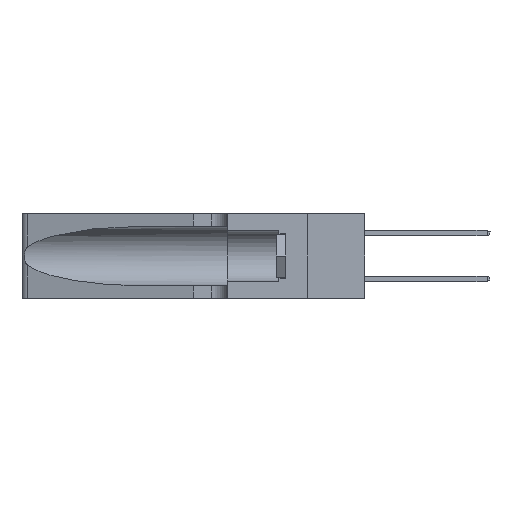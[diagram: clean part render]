
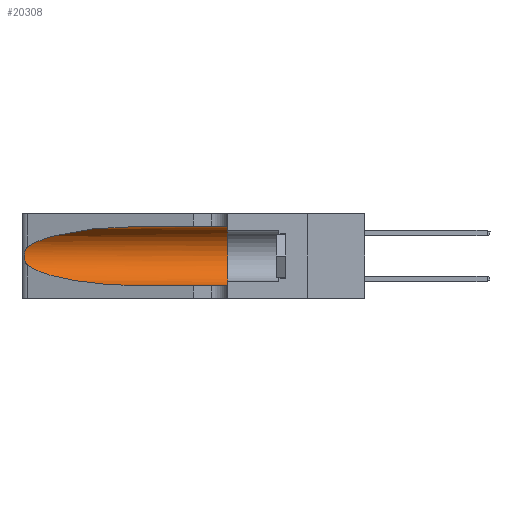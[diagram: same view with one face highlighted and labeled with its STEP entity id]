
A CAD part, left-side view. The second image highlights one B-rep face of the part: STEP entity #20308.
In plain terms, the highlighted cylindrical face has radius 3.308 mm (diameter 6.617 mm), a partial arc.
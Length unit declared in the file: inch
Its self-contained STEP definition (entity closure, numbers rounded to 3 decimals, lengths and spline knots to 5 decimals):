
#182 = CARTESIAN_POINT ( 'NONE',  ( 0.25639, 1.23184, 0.21858 ) ) ;
#560 = DIRECTION ( 'NONE',  ( 0., -1., 0. ) ) ;
#1215 = EDGE_CURVE ( 'NONE', #14818, #31055, #26149, .T. ) ;
#1867 = CARTESIAN_POINT ( 'NONE',  ( 0.1305, 0.72297, 0.05475 ) ) ;
#2061 = ORIENTED_EDGE ( 'NONE', *, *, #29288, .T. ) ;
#2638 = CARTESIAN_POINT ( 'NONE',  ( 0.25856, 1.23593, 0.16098 ) ) ;
#3086 = CARTESIAN_POINT ( 'NONE',  ( 0.1305, 0.72297, 0.05475 ) ) ;
#3107 = EDGE_CURVE ( 'NONE', #6114, #22241, #11570, .T. ) ;
#3572 = EDGE_LOOP ( 'NONE', ( #2061, #31905, #7103, #6359, #7499, #11759 ) ) ;
#5109 = CARTESIAN_POINT ( 'NONE',  ( 0.25555, 1.22993, 0.14849 ) ) ;
#5415 = CARTESIAN_POINT ( 'NONE',  ( 0.25487, 1.22718, 0.22369 ) ) ;
#5773 = EDGE_CURVE ( 'NONE', #16697, #6114, #20204, .T. ) ;
#5840 = FACE_OUTER_BOUND ( 'NONE', #3572, .T. ) ;
#6114 = VERTEX_POINT ( 'NONE', #25859 ) ;
#6311 = AXIS2_PLACEMENT_3D ( 'NONE', #24553, #15568, #17398 ) ;
#6359 = ORIENTED_EDGE ( 'NONE', *, *, #10248, .T. ) ;
#6802 = CARTESIAN_POINT ( 'NONE',  ( 0.1305, 0.72297, 0.31525 ) ) ;
#7103 = ORIENTED_EDGE ( 'NONE', *, *, #3107, .T. ) ;
#7499 = ORIENTED_EDGE ( 'NONE', *, *, #1215, .F. ) ;
#7615 = CARTESIAN_POINT ( 'NONE',  ( 0.25487, 1.22718, 0.14631 ) ) ;
#10207 = CARTESIAN_POINT ( 'NONE',  ( 0.1305, 0.35, 0.05475 ) ) ;
#10248 = EDGE_CURVE ( 'NONE', #22241, #31055, #28049, .T. ) ;
#10265 = CARTESIAN_POINT ( 'NONE',  ( 0.25787, 1.23484, 0.2124 ) ) ;
#10370 = CARTESIAN_POINT ( 'NONE',  ( 0.26075, 1.23896, 0.178 ) ) ;
#10415 = CARTESIAN_POINT ( 'NONE',  ( 0.1305, 0.72297, 0.31525 ) ) ;
#10832 = LINE ( 'NONE', #13184, #22424 ) ;
#11570 =( BOUNDED_CURVE ( )  B_SPLINE_CURVE ( 3, ( #19028, #19250, #26497, #1867 ),
 .UNSPECIFIED., .F., .F. ) 
 B_SPLINE_CURVE_WITH_KNOTS ( ( 4, 4 ),
 ( 3.44316, 4.71239 ),
 .UNSPECIFIED. ) 
 CURVE ( )  GEOMETRIC_REPRESENTATION_ITEM ( )  RATIONAL_B_SPLINE_CURVE ( ( 1., 0.87, 0.87, 1. ) ) 
 REPRESENTATION_ITEM ( '' )  );
#11759 = ORIENTED_EDGE ( 'NONE', *, *, #20320, .F. ) ;
#12195 = DIRECTION ( 'NONE',  ( 0., 1., 0. ) ) ;
#12853 = CARTESIAN_POINT ( 'NONE',  ( 0.1305, 1.61858, 0.05475 ) ) ;
#13184 = CARTESIAN_POINT ( 'NONE',  ( 0.1305, 1.61858, 0.31525 ) ) ;
#13583 = AXIS2_PLACEMENT_3D ( 'NONE', #14781, #12195, #29598 ) ;
#14527 =( BOUNDED_CURVE ( )  B_SPLINE_CURVE ( 3, ( #10415, #22418, #28750, #14672 ),
 .UNSPECIFIED., .F., .F. ) 
 B_SPLINE_CURVE_WITH_KNOTS ( ( 4, 4 ),
 ( 1.5708, 2.84003 ),
 .UNSPECIFIED. ) 
 CURVE ( )  GEOMETRIC_REPRESENTATION_ITEM ( )  RATIONAL_B_SPLINE_CURVE ( ( 1., 0.87, 0.87, 1. ) ) 
 REPRESENTATION_ITEM ( '' )  );
#14672 = CARTESIAN_POINT ( 'NONE',  ( 0.25487, 1.22718, 0.22369 ) ) ;
#14781 = CARTESIAN_POINT ( 'NONE',  ( 0.1305, 0.35, 0.185 ) ) ;
#14818 = VERTEX_POINT ( 'NONE', #25542 ) ;
#15047 = CARTESIAN_POINT ( 'NONE',  ( 0.25854, 1.2359, 0.20912 ) ) ;
#15568 = DIRECTION ( 'NONE',  ( 0., -1., 0. ) ) ;
#16697 = VERTEX_POINT ( 'NONE', #29716 ) ;
#17398 = DIRECTION ( 'NONE',  ( 0., 0., -1. ) ) ;
#17439 = CARTESIAN_POINT ( 'NONE',  ( 0.26018, 1.23835, 0.19895 ) ) ;
#17639 = CARTESIAN_POINT ( 'NONE',  ( 0.26075, 1.23896, 0.19203 ) ) ;
#17830 = DIRECTION ( 'NONE',  ( 0., -1., 0. ) ) ;
#19028 = CARTESIAN_POINT ( 'NONE',  ( 0.25487, 1.22718, 0.14631 ) ) ;
#19250 = CARTESIAN_POINT ( 'NONE',  ( 0.2373, 1.15595, 0.08982 ) ) ;
#20125 = CARTESIAN_POINT ( 'NONE',  ( 0.25789, 1.23486, 0.15765 ) ) ;
#20204 = B_SPLINE_CURVE_WITH_KNOTS ( 'NONE', 3,
 ( #5415, #22681, #182, #10265, #15047, #17439, #17639, #10370, #24993, #2638, #20125, #27611, #5109, #7615 ),
 .UNSPECIFIED., .F., .F.,
 ( 4, 2, 2, 2, 2, 2, 4 ),
 ( 0., 0.00027, 0.00053, 0.00107, 0.0016, 0.00187, 0.00214 ),
 .UNSPECIFIED. ) ;
#20308 = ADVANCED_FACE ( 'NONE', ( #5840 ), #28262, .F. ) ;
#20320 = EDGE_CURVE ( 'NONE', #25847, #14818, #10832, .T. ) ;
#22241 = VERTEX_POINT ( 'NONE', #3086 ) ;
#22418 = CARTESIAN_POINT ( 'NONE',  ( 0.18966, 0.96281, 0.31525 ) ) ;
#22424 = VECTOR ( 'NONE', #560, 39.37008 ) ;
#22681 = CARTESIAN_POINT ( 'NONE',  ( 0.25555, 1.22994, 0.2215 ) ) ;
#24553 = CARTESIAN_POINT ( 'NONE',  ( 0.1305, 1.61858, 0.185 ) ) ;
#24993 = CARTESIAN_POINT ( 'NONE',  ( 0.26017, 1.23833, 0.17102 ) ) ;
#25542 = CARTESIAN_POINT ( 'NONE',  ( 0.1305, 0.35, 0.31525 ) ) ;
#25678 = VECTOR ( 'NONE', #17830, 39.37008 ) ;
#25847 = VERTEX_POINT ( 'NONE', #6802 ) ;
#25859 = CARTESIAN_POINT ( 'NONE',  ( 0.25487, 1.22718, 0.14631 ) ) ;
#26149 = CIRCLE ( 'NONE', #13583, 0.13025 ) ;
#26497 = CARTESIAN_POINT ( 'NONE',  ( 0.18966, 0.96281, 0.05475 ) ) ;
#27611 = CARTESIAN_POINT ( 'NONE',  ( 0.25639, 1.23186, 0.15144 ) ) ;
#28049 = LINE ( 'NONE', #12853, #25678 ) ;
#28262 = CYLINDRICAL_SURFACE ( 'NONE', #6311, 0.13025 ) ;
#28750 = CARTESIAN_POINT ( 'NONE',  ( 0.2373, 1.15595, 0.28018 ) ) ;
#29288 = EDGE_CURVE ( 'NONE', #25847, #16697, #14527, .T. ) ;
#29598 = DIRECTION ( 'NONE',  ( 0., 0., 1. ) ) ;
#29716 = CARTESIAN_POINT ( 'NONE',  ( 0.25487, 1.22718, 0.22369 ) ) ;
#31055 = VERTEX_POINT ( 'NONE', #10207 ) ;
#31905 = ORIENTED_EDGE ( 'NONE', *, *, #5773, .T. ) ;
